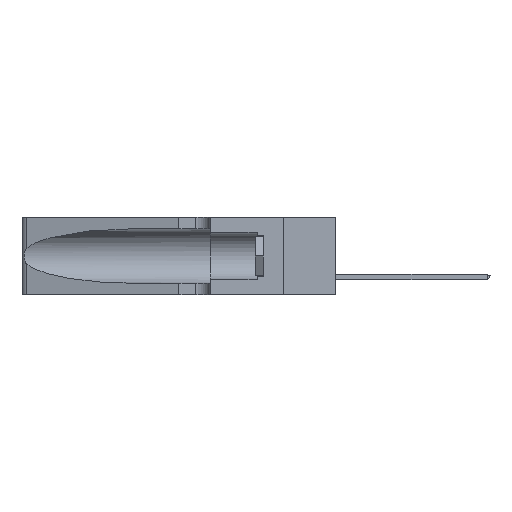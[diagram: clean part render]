
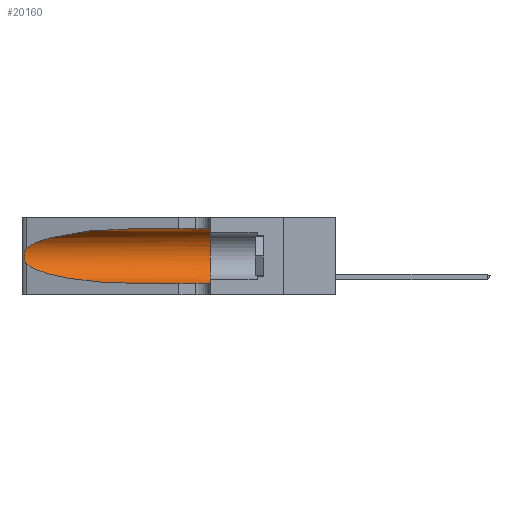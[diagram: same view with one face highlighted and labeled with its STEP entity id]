
A CAD part, left-side view. The second image highlights one B-rep face of the part: STEP entity #20160.
In plain terms, the highlighted cylindrical face has radius 3.308 mm (diameter 6.617 mm), a partial arc.
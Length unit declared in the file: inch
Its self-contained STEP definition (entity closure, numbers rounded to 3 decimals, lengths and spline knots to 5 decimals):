
#189 = CARTESIAN_POINT ( 'NONE',  ( 0.25487, 1.22718, 0.22369 ) ) ;
#567 =( BOUNDED_CURVE ( )  B_SPLINE_CURVE ( 3, ( #21067, #11496, #33908, #24511 ),
 .UNSPECIFIED., .F., .F. ) 
 B_SPLINE_CURVE_WITH_KNOTS ( ( 4, 4 ),
 ( 3.44316, 4.71239 ),
 .UNSPECIFIED. ) 
 CURVE ( )  GEOMETRIC_REPRESENTATION_ITEM ( )  RATIONAL_B_SPLINE_CURVE ( ( 1., 0.87, 0.87, 1. ) ) 
 REPRESENTATION_ITEM ( '' )  );
#1320 = ORIENTED_EDGE ( 'NONE', *, *, #39031, .T. ) ;
#1651 = CARTESIAN_POINT ( 'NONE',  ( 0.25487, 1.22718, 0.22369 ) ) ;
#1917 = CARTESIAN_POINT ( 'NONE',  ( 0.25555, 1.22993, 0.14849 ) ) ;
#2857 = EDGE_CURVE ( 'NONE', #33533, #32106, #4764, .T. ) ;
#2914 = EDGE_CURVE ( 'NONE', #14589, #8901, #31468, .T. ) ;
#2948 = DIRECTION ( 'NONE',  ( 0., -1., 0. ) ) ;
#3503 = CARTESIAN_POINT ( 'NONE',  ( 0.1305, 0.35, 0.05475 ) ) ;
#3843 = AXIS2_PLACEMENT_3D ( 'NONE', #5301, #21085, #27400 ) ;
#4764 = CIRCLE ( 'NONE', #36935, 0.13025 ) ;
#5301 = CARTESIAN_POINT ( 'NONE',  ( 0.1305, 1.61858, 0.185 ) ) ;
#5535 = CARTESIAN_POINT ( 'NONE',  ( 0.1305, 1.61858, 0.05475 ) ) ;
#7893 = CARTESIAN_POINT ( 'NONE',  ( 0.25639, 1.23184, 0.21858 ) ) ;
#8737 = FACE_OUTER_BOUND ( 'NONE', #37835, .T. ) ;
#8901 = VERTEX_POINT ( 'NONE', #12028 ) ;
#9352 = CARTESIAN_POINT ( 'NONE',  ( 0.18966, 0.96281, 0.31525 ) ) ;
#10817 = DIRECTION ( 'NONE',  ( 0., 1., 0. ) ) ;
#10891 =( BOUNDED_CURVE ( )  B_SPLINE_CURVE ( 3, ( #15809, #9352, #37716, #189 ),
 .UNSPECIFIED., .F., .T. ) 
 B_SPLINE_CURVE_WITH_KNOTS ( ( 4, 4 ),
 ( 1.5708, 2.84003 ),
 .UNSPECIFIED. ) 
 CURVE ( )  GEOMETRIC_REPRESENTATION_ITEM ( )  RATIONAL_B_SPLINE_CURVE ( ( 1., 0.87, 0.87, 1. ) ) 
 REPRESENTATION_ITEM ( '' )  );
#11116 = CARTESIAN_POINT ( 'NONE',  ( 0.25787, 1.23484, 0.2124 ) ) ;
#11496 = CARTESIAN_POINT ( 'NONE',  ( 0.2373, 1.15595, 0.08982 ) ) ;
#11886 = DIRECTION ( 'NONE',  ( 0., -1., 0. ) ) ;
#12028 = CARTESIAN_POINT ( 'NONE',  ( 0.25487, 1.22718, 0.14631 ) ) ;
#13752 = ORIENTED_EDGE ( 'NONE', *, *, #2857, .F. ) ;
#14589 = VERTEX_POINT ( 'NONE', #26853 ) ;
#14702 = VECTOR ( 'NONE', #2948, 39.37008 ) ;
#14906 = VERTEX_POINT ( 'NONE', #20835 ) ;
#15265 = ORIENTED_EDGE ( 'NONE', *, *, #33692, .T. ) ;
#15341 = EDGE_CURVE ( 'NONE', #14906, #33533, #31349, .T. ) ;
#15809 = CARTESIAN_POINT ( 'NONE',  ( 0.1305, 0.72297, 0.31525 ) ) ;
#17246 = CARTESIAN_POINT ( 'NONE',  ( 0.26075, 1.23896, 0.178 ) ) ;
#17802 = CARTESIAN_POINT ( 'NONE',  ( 0.25487, 1.22718, 0.14631 ) ) ;
#20160 = ADVANCED_FACE ( 'NONE', ( #8737 ), #35703, .F. ) ;
#20549 = CARTESIAN_POINT ( 'NONE',  ( 0.26018, 1.23835, 0.19895 ) ) ;
#20704 = ORIENTED_EDGE ( 'NONE', *, *, #36017, .T. ) ;
#20835 = CARTESIAN_POINT ( 'NONE',  ( 0.1305, 0.72297, 0.31525 ) ) ;
#20938 = ORIENTED_EDGE ( 'NONE', *, *, #15341, .F. ) ;
#21067 = CARTESIAN_POINT ( 'NONE',  ( 0.25487, 1.22718, 0.14631 ) ) ;
#21085 = DIRECTION ( 'NONE',  ( 0., -1., 0. ) ) ;
#22119 = VECTOR ( 'NONE', #11886, 39.37008 ) ;
#23451 = CARTESIAN_POINT ( 'NONE',  ( 0.25555, 1.22994, 0.2215 ) ) ;
#23734 = CARTESIAN_POINT ( 'NONE',  ( 0.25856, 1.23593, 0.16098 ) ) ;
#24511 = CARTESIAN_POINT ( 'NONE',  ( 0.1305, 0.72297, 0.05475 ) ) ;
#26853 = CARTESIAN_POINT ( 'NONE',  ( 0.25487, 1.22718, 0.22369 ) ) ;
#27400 = DIRECTION ( 'NONE',  ( 0., 0., -1. ) ) ;
#28676 = CARTESIAN_POINT ( 'NONE',  ( 0.1305, 0.35, 0.31525 ) ) ;
#29733 = ORIENTED_EDGE ( 'NONE', *, *, #2914, .T. ) ;
#30018 = CARTESIAN_POINT ( 'NONE',  ( 0.1305, 0.35, 0.185 ) ) ;
#31349 = LINE ( 'NONE', #38238, #14702 ) ;
#31399 = LINE ( 'NONE', #5535, #22119 ) ;
#31468 = B_SPLINE_CURVE_WITH_KNOTS ( 'NONE', 3,
 ( #1651, #23451, #7893, #11116, #36129, #20549, #35985, #17246, #39300, #23734, #33135, #38884, #1917, #17802 ),
 .UNSPECIFIED., .F., .F.,
 ( 4, 2, 2, 2, 2, 2, 4 ),
 ( 0., 0.00027, 0.00053, 0.00107, 0.0016, 0.00187, 0.00214 ),
 .UNSPECIFIED. ) ;
#32106 = VERTEX_POINT ( 'NONE', #3503 ) ;
#32853 = VERTEX_POINT ( 'NONE', #35441 ) ;
#33135 = CARTESIAN_POINT ( 'NONE',  ( 0.25789, 1.23486, 0.15765 ) ) ;
#33533 = VERTEX_POINT ( 'NONE', #28676 ) ;
#33692 = EDGE_CURVE ( 'NONE', #8901, #32853, #567, .T. ) ;
#33908 = CARTESIAN_POINT ( 'NONE',  ( 0.18966, 0.96281, 0.05475 ) ) ;
#35441 = CARTESIAN_POINT ( 'NONE',  ( 0.1305, 0.72297, 0.05475 ) ) ;
#35703 = CYLINDRICAL_SURFACE ( 'NONE', #3843, 0.13025 ) ;
#35985 = CARTESIAN_POINT ( 'NONE',  ( 0.26075, 1.23896, 0.19203 ) ) ;
#36017 = EDGE_CURVE ( 'NONE', #32853, #32106, #31399, .T. ) ;
#36129 = CARTESIAN_POINT ( 'NONE',  ( 0.25854, 1.2359, 0.20912 ) ) ;
#36935 = AXIS2_PLACEMENT_3D ( 'NONE', #30018, #10817, #39159 ) ;
#37716 = CARTESIAN_POINT ( 'NONE',  ( 0.2373, 1.15595, 0.28018 ) ) ;
#37835 = EDGE_LOOP ( 'NONE', ( #1320, #29733, #15265, #20704, #13752, #20938 ) ) ;
#38238 = CARTESIAN_POINT ( 'NONE',  ( 0.1305, 1.61858, 0.31525 ) ) ;
#38884 = CARTESIAN_POINT ( 'NONE',  ( 0.25639, 1.23186, 0.15144 ) ) ;
#39031 = EDGE_CURVE ( 'NONE', #14906, #14589, #10891, .T. ) ;
#39159 = DIRECTION ( 'NONE',  ( 0., 0., 1. ) ) ;
#39300 = CARTESIAN_POINT ( 'NONE',  ( 0.26017, 1.23833, 0.17102 ) ) ;
